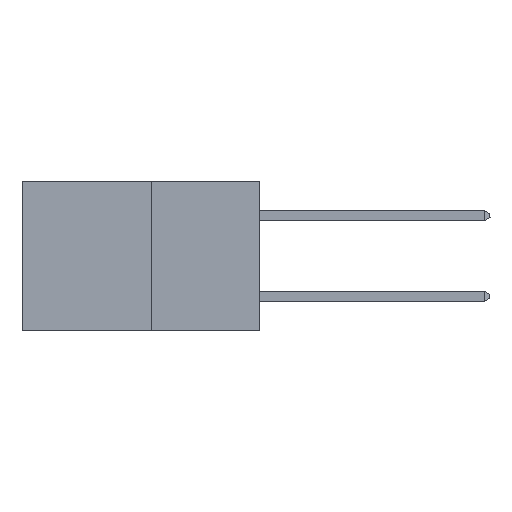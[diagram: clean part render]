
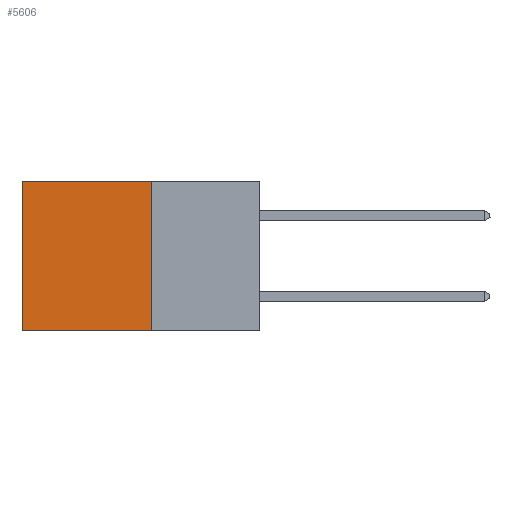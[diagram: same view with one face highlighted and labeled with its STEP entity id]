
A CAD part, left-side view. The second image highlights one B-rep face of the part: STEP entity #5606.
In plain terms, the highlighted planar face has unit normal (-1, 0, 0).
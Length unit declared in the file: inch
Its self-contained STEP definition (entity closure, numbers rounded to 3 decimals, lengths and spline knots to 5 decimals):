
#594 = VECTOR ( 'NONE', #7328, 39.37008 ) ;
#632 = DIRECTION ( 'NONE',  ( 0., 0., -1. ) ) ;
#662 = DIRECTION ( 'NONE',  ( 1., 0., 0. ) ) ;
#666 = CARTESIAN_POINT ( 'NONE',  ( 0.277, 0.59, -0.37 ) ) ;
#669 = ORIENTED_EDGE ( 'NONE', *, *, #3339, .F. ) ;
#777 = LINE ( 'NONE', #5942, #6353 ) ;
#792 = PLANE ( 'NONE',  #1644 ) ;
#837 = LINE ( 'NONE', #6714, #594 ) ;
#912 = DIRECTION ( 'NONE',  ( 0., 0., -1. ) ) ;
#1092 = CARTESIAN_POINT ( 'NONE',  ( 0.277, 0.27, -0.37 ) ) ;
#1190 = CARTESIAN_POINT ( 'NONE',  ( 0.277, 0.27, -0.37 ) ) ;
#1644 = AXIS2_PLACEMENT_3D ( 'NONE', #1092, #662, #632 ) ;
#1919 = EDGE_CURVE ( 'NONE', #6951, #8172, #8400, .T. ) ;
#2018 = LINE ( 'NONE', #1190, #7572 ) ;
#2260 = VERTEX_POINT ( 'NONE', #5802 ) ;
#2411 = FACE_OUTER_BOUND ( 'NONE', #3255, .T. ) ;
#2587 = VECTOR ( 'NONE', #912, 39.37008 ) ;
#2604 = ORIENTED_EDGE ( 'NONE', *, *, #5376, .F. ) ;
#3255 = EDGE_LOOP ( 'NONE', ( #6237, #2604, #669, #6485 ) ) ;
#3339 = EDGE_CURVE ( 'NONE', #7917, #2260, #2018, .T. ) ;
#3561 = CARTESIAN_POINT ( 'NONE',  ( 0.277, 0.59, -0.37 ) ) ;
#5376 = EDGE_CURVE ( 'NONE', #2260, #8172, #837, .T. ) ;
#5547 = CARTESIAN_POINT ( 'NONE',  ( 0.277, 0.27, 0. ) ) ;
#5606 = ADVANCED_FACE ( 'NONE', ( #2411 ), #792, .F. ) ;
#5802 = CARTESIAN_POINT ( 'NONE',  ( 0.277, 0.27, -0.37 ) ) ;
#5942 = CARTESIAN_POINT ( 'NONE',  ( 0.277, 0.27, 0. ) ) ;
#6204 = CARTESIAN_POINT ( 'NONE',  ( 0.277, 0.59, 0. ) ) ;
#6237 = ORIENTED_EDGE ( 'NONE', *, *, #1919, .T. ) ;
#6353 = VECTOR ( 'NONE', #8113, 39.37008 ) ;
#6485 = ORIENTED_EDGE ( 'NONE', *, *, #8382, .T. ) ;
#6714 = CARTESIAN_POINT ( 'NONE',  ( 0.277, 0.27, -0.37 ) ) ;
#6951 = VERTEX_POINT ( 'NONE', #6204 ) ;
#7328 = DIRECTION ( 'NONE',  ( 0., 1., 0. ) ) ;
#7572 = VECTOR ( 'NONE', #9174, 39.37008 ) ;
#7917 = VERTEX_POINT ( 'NONE', #5547 ) ;
#8113 = DIRECTION ( 'NONE',  ( 0., 1., 0. ) ) ;
#8172 = VERTEX_POINT ( 'NONE', #3561 ) ;
#8382 = EDGE_CURVE ( 'NONE', #7917, #6951, #777, .T. ) ;
#8400 = LINE ( 'NONE', #666, #2587 ) ;
#9174 = DIRECTION ( 'NONE',  ( 0., 0., -1. ) ) ;
